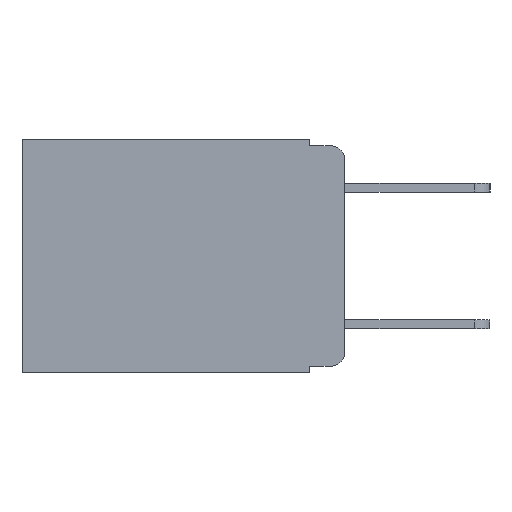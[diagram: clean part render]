
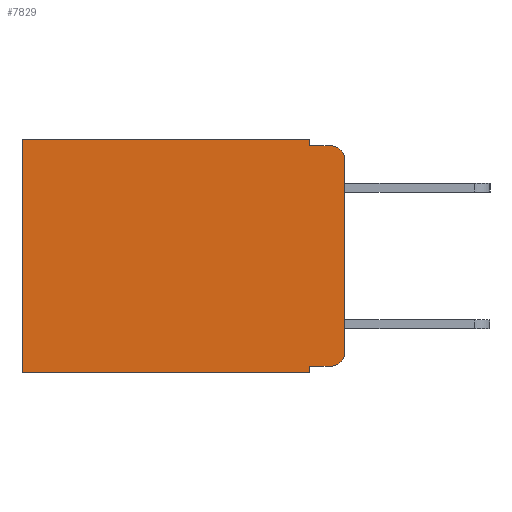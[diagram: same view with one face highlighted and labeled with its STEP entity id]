
A CAD part, left-side view. The second image highlights one B-rep face of the part: STEP entity #7829.
In plain terms, the highlighted planar face has unit normal (-1, 0, 0).
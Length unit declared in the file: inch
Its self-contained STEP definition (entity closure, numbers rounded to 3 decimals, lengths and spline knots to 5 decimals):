
#115 = VERTEX_POINT ( 'NONE', #9444 ) ;
#183 = AXIS2_PLACEMENT_3D ( 'NONE', #2190, #2118, #1999 ) ;
#326 = EDGE_CURVE ( 'NONE', #11521, #2083, #1393, .T. ) ;
#895 = VECTOR ( 'NONE', #9134, 39.37008 ) ;
#930 = VERTEX_POINT ( 'NONE', #8988 ) ;
#1213 = EDGE_CURVE ( 'NONE', #4807, #11521, #2537, .T. ) ;
#1242 = EDGE_CURVE ( 'NONE', #930, #2083, #5583, .T. ) ;
#1247 = EDGE_CURVE ( 'NONE', #13590, #13474, #1576, .T. ) ;
#1326 = CARTESIAN_POINT ( 'NONE',  ( 0.298, 0.051, -0.01 ) ) ;
#1393 = LINE ( 'NONE', #8176, #895 ) ;
#1501 = EDGE_CURVE ( 'NONE', #115, #3274, #1814, .T. ) ;
#1504 = CARTESIAN_POINT ( 'NONE',  ( 0.298, 0.473, 0. ) ) ;
#1576 = LINE ( 'NONE', #16256, #9026 ) ;
#1704 = CARTESIAN_POINT ( 'NONE',  ( 0.298, 0.051, -0.333 ) ) ;
#1814 = CIRCLE ( 'NONE', #3340, 0.02 ) ;
#1924 = DIRECTION ( 'NONE',  ( -1., 0., 0. ) ) ;
#1999 = DIRECTION ( 'NONE',  ( 0., 0., -1. ) ) ;
#2083 = VERTEX_POINT ( 'NONE', #8828 ) ;
#2118 = DIRECTION ( 'NONE',  ( -1., 0., 0. ) ) ;
#2158 = CARTESIAN_POINT ( 'NONE',  ( 0.298, 0.02, -0.313 ) ) ;
#2190 = CARTESIAN_POINT ( 'NONE',  ( 0.298, 0.02, -0.03 ) ) ;
#2537 = LINE ( 'NONE', #16332, #16696 ) ;
#2655 = ORIENTED_EDGE ( 'NONE', *, *, #3888, .T. ) ;
#2782 = CARTESIAN_POINT ( 'NONE',  ( 0.298, 0.051, 0. ) ) ;
#3274 = VERTEX_POINT ( 'NONE', #4617 ) ;
#3340 = AXIS2_PLACEMENT_3D ( 'NONE', #2158, #1924, #9384 ) ;
#3524 = EDGE_CURVE ( 'NONE', #4745, #3274, #11580, .T. ) ;
#3773 = VECTOR ( 'NONE', #8461, 39.37008 ) ;
#3808 = EDGE_CURVE ( 'NONE', #4745, #4594, #12593, .T. ) ;
#3831 = EDGE_LOOP ( 'NONE', ( #6440, #14867, #4275, #17481, #13471, #14158, #14907, #16106, #2655, #5018 ) ) ;
#3864 = EDGE_CURVE ( 'NONE', #13474, #4594, #8633, .T. ) ;
#3888 = EDGE_CURVE ( 'NONE', #4807, #115, #4166, .T. ) ;
#4166 = LINE ( 'NONE', #8877, #14647 ) ;
#4275 = ORIENTED_EDGE ( 'NONE', *, *, #3864, .F. ) ;
#4364 = DIRECTION ( 'NONE',  ( 0., 0., -1. ) ) ;
#4594 = VERTEX_POINT ( 'NONE', #11792 ) ;
#4617 = CARTESIAN_POINT ( 'NONE',  ( 0.298, 0., -0.313 ) ) ;
#4745 = VERTEX_POINT ( 'NONE', #5745 ) ;
#4807 = VERTEX_POINT ( 'NONE', #1704 ) ;
#5018 = ORIENTED_EDGE ( 'NONE', *, *, #1501, .T. ) ;
#5583 = LINE ( 'NONE', #1504, #15654 ) ;
#5623 = CARTESIAN_POINT ( 'NONE',  ( 0.298, 0.051, -0.01 ) ) ;
#5745 = CARTESIAN_POINT ( 'NONE',  ( 0.298, 0., -0.03 ) ) ;
#6440 = ORIENTED_EDGE ( 'NONE', *, *, #3524, .F. ) ;
#6483 = DIRECTION ( 'NONE',  ( 0., 0., -1. ) ) ;
#7001 = CARTESIAN_POINT ( 'NONE',  ( 0.298, 0., 0. ) ) ;
#7483 = PLANE ( 'NONE',  #14646 ) ;
#7829 = ADVANCED_FACE ( 'NONE', ( #13303 ), #7483, .F. ) ;
#8176 = CARTESIAN_POINT ( 'NONE',  ( 0.298, 0., -0.343 ) ) ;
#8461 = DIRECTION ( 'NONE',  ( 0., 1., 0. ) ) ;
#8633 = LINE ( 'NONE', #1326, #15001 ) ;
#8828 = CARTESIAN_POINT ( 'NONE',  ( 0.298, 0.473, -0.343 ) ) ;
#8832 = DIRECTION ( 'NONE',  ( 0., -1., 0. ) ) ;
#8877 = CARTESIAN_POINT ( 'NONE',  ( 0.298, 0.051, -0.333 ) ) ;
#8921 = DIRECTION ( 'NONE',  ( 0., 0., -1. ) ) ;
#8988 = CARTESIAN_POINT ( 'NONE',  ( 0.298, 0.473, 0. ) ) ;
#9026 = VECTOR ( 'NONE', #4364, 39.37008 ) ;
#9134 = DIRECTION ( 'NONE',  ( 0., 1., 0. ) ) ;
#9384 = DIRECTION ( 'NONE',  ( 0., 0., -1. ) ) ;
#9444 = CARTESIAN_POINT ( 'NONE',  ( 0.298, 0.02, -0.333 ) ) ;
#11167 = VECTOR ( 'NONE', #6483, 39.37008 ) ;
#11521 = VERTEX_POINT ( 'NONE', #12957 ) ;
#11544 = CARTESIAN_POINT ( 'NONE',  ( 0.298, 0., 0. ) ) ;
#11580 = LINE ( 'NONE', #14663, #11167 ) ;
#11792 = CARTESIAN_POINT ( 'NONE',  ( 0.298, 0.02, -0.01 ) ) ;
#12238 = DIRECTION ( 'NONE',  ( 0., -1., 0. ) ) ;
#12593 = CIRCLE ( 'NONE', #183, 0.02 ) ;
#12957 = CARTESIAN_POINT ( 'NONE',  ( 0.298, 0.051, -0.343 ) ) ;
#13033 = DIRECTION ( 'NONE',  ( 0., 0., -1. ) ) ;
#13303 = FACE_OUTER_BOUND ( 'NONE', #3831, .T. ) ;
#13471 = ORIENTED_EDGE ( 'NONE', *, *, #17247, .T. ) ;
#13474 = VERTEX_POINT ( 'NONE', #5623 ) ;
#13590 = VERTEX_POINT ( 'NONE', #2782 ) ;
#13893 = DIRECTION ( 'NONE',  ( 0., 0., -1. ) ) ;
#14158 = ORIENTED_EDGE ( 'NONE', *, *, #1242, .T. ) ;
#14646 = AXIS2_PLACEMENT_3D ( 'NONE', #11544, #16313, #8921 ) ;
#14647 = VECTOR ( 'NONE', #8832, 39.37008 ) ;
#14663 = CARTESIAN_POINT ( 'NONE',  ( 0.298, 0., 0. ) ) ;
#14712 = LINE ( 'NONE', #7001, #3773 ) ;
#14867 = ORIENTED_EDGE ( 'NONE', *, *, #3808, .T. ) ;
#14907 = ORIENTED_EDGE ( 'NONE', *, *, #326, .F. ) ;
#15001 = VECTOR ( 'NONE', #12238, 39.37008 ) ;
#15654 = VECTOR ( 'NONE', #13033, 39.37008 ) ;
#16106 = ORIENTED_EDGE ( 'NONE', *, *, #1213, .F. ) ;
#16256 = CARTESIAN_POINT ( 'NONE',  ( 0.298, 0.051, 0. ) ) ;
#16313 = DIRECTION ( 'NONE',  ( 1., 0., 0. ) ) ;
#16332 = CARTESIAN_POINT ( 'NONE',  ( 0.298, 0.051, 0. ) ) ;
#16696 = VECTOR ( 'NONE', #13893, 39.37008 ) ;
#17247 = EDGE_CURVE ( 'NONE', #13590, #930, #14712, .T. ) ;
#17481 = ORIENTED_EDGE ( 'NONE', *, *, #1247, .F. ) ;
